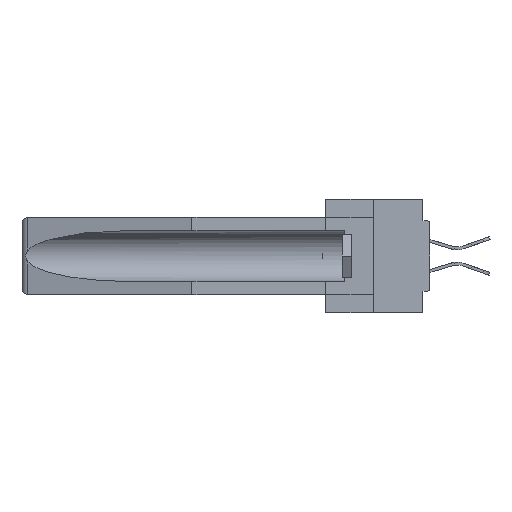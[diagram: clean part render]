
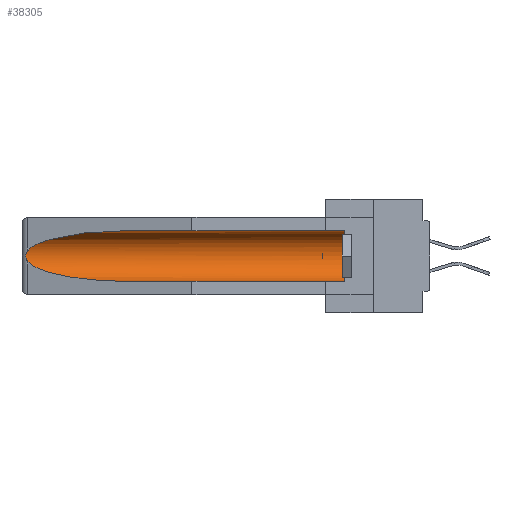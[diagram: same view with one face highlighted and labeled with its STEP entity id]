
A CAD part, left-side view. The second image highlights one B-rep face of the part: STEP entity #38305.
In plain terms, the highlighted cylindrical face has radius 2.857 mm (diameter 5.715 mm), a partial arc.
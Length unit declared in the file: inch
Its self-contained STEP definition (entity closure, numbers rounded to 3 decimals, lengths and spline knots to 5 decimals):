
#149 =( BOUNDED_CURVE ( )  B_SPLINE_CURVE ( 3, ( #30174, #41840, #18951, #27632 ),
 .UNSPECIFIED., .F., .F. ) 
 B_SPLINE_CURVE_WITH_KNOTS ( ( 4, 4 ),
 ( 4.71239, 6.08839 ),
 .UNSPECIFIED. ) 
 CURVE ( )  GEOMETRIC_REPRESENTATION_ITEM ( )  RATIONAL_B_SPLINE_CURVE ( ( 1., 0.848, 0.848, 1. ) ) 
 REPRESENTATION_ITEM ( '' )  );
#609 = VECTOR ( 'NONE', #40306, 39.37008 ) ;
#1853 = CARTESIAN_POINT ( 'NONE',  ( 0.2675, 1.53308, -0.16763 ) ) ;
#1897 = AXIS2_PLACEMENT_3D ( 'NONE', #40304, #32116, #47619 ) ;
#2174 = CARTESIAN_POINT ( 'NONE',  ( 0.26655, 1.53094, -0.18657 ) ) ;
#3349 = ORIENTED_EDGE ( 'NONE', *, *, #41865, .F. ) ;
#3635 = EDGE_CURVE ( 'NONE', #12110, #45306, #10200, .T. ) ;
#4641 = CARTESIAN_POINT ( 'NONE',  ( 0.26537, 1.52718, -0.19328 ) ) ;
#7684 = EDGE_CURVE ( 'NONE', #45306, #15028, #149, .T. ) ;
#9271 = CARTESIAN_POINT ( 'NONE',  ( 0.155, 0.126, -0.284 ) ) ;
#10200 = LINE ( 'NONE', #21074, #609 ) ;
#12110 = VERTEX_POINT ( 'NONE', #32921 ) ;
#12391 = CARTESIAN_POINT ( 'NONE',  ( 0.155, 1.07973, -0.059 ) ) ;
#13358 = CARTESIAN_POINT ( 'NONE',  ( 0.2673, 1.53269, -0.17917 ) ) ;
#13487 = DIRECTION ( 'NONE',  ( 0., 1., 0. ) ) ;
#13700 = CARTESIAN_POINT ( 'NONE',  ( 0.26597, 1.52961, -0.15275 ) ) ;
#15028 = VERTEX_POINT ( 'NONE', #18644 ) ;
#16004 = CARTESIAN_POINT ( 'NONE',  ( 0.155, -0.30754, -0.284 ) ) ;
#16397 = ORIENTED_EDGE ( 'NONE', *, *, #33899, .T. ) ;
#16442 =( BOUNDED_CURVE ( )  B_SPLINE_CURVE ( 3, ( #19342, #23220, #18688, #26744 ),
 .UNSPECIFIED., .F., .F. ) 
 B_SPLINE_CURVE_WITH_KNOTS ( ( 4, 4 ),
 ( 0.1948, 1.5708 ),
 .UNSPECIFIED. ) 
 CURVE ( )  GEOMETRIC_REPRESENTATION_ITEM ( )  RATIONAL_B_SPLINE_CURVE ( ( 1., 0.848, 0.848, 1. ) ) 
 REPRESENTATION_ITEM ( '' )  );
#17885 = ORIENTED_EDGE ( 'NONE', *, *, #40342, .T. ) ;
#18644 = CARTESIAN_POINT ( 'NONE',  ( 0.26537, 1.52718, -0.14972 ) ) ;
#18688 = CARTESIAN_POINT ( 'NONE',  ( 0.21114, 1.30732, -0.284 ) ) ;
#18951 = CARTESIAN_POINT ( 'NONE',  ( 0.25451, 1.48313, -0.09465 ) ) ;
#19236 = VERTEX_POINT ( 'NONE', #4641 ) ;
#19342 = CARTESIAN_POINT ( 'NONE',  ( 0.26537, 1.52718, -0.19328 ) ) ;
#20129 = CIRCLE ( 'NONE', #1897, 0.1125 ) ;
#21074 = CARTESIAN_POINT ( 'NONE',  ( 0.155, -0.30754, -0.059 ) ) ;
#23220 = CARTESIAN_POINT ( 'NONE',  ( 0.25451, 1.48313, -0.24835 ) ) ;
#23556 = ORIENTED_EDGE ( 'NONE', *, *, #29662, .T. ) ;
#23652 = ORIENTED_EDGE ( 'NONE', *, *, #3635, .T. ) ;
#24253 = ORIENTED_EDGE ( 'NONE', *, *, #7684, .T. ) ;
#25158 = AXIS2_PLACEMENT_3D ( 'NONE', #40441, #13487, #47932 ) ;
#26744 = CARTESIAN_POINT ( 'NONE',  ( 0.155, 1.07973, -0.284 ) ) ;
#27632 = CARTESIAN_POINT ( 'NONE',  ( 0.26537, 1.52718, -0.14972 ) ) ;
#28127 = CYLINDRICAL_SURFACE ( 'NONE', #25158, 0.1125 ) ;
#28968 = CARTESIAN_POINT ( 'NONE',  ( 0.26597, 1.5296, -0.19026 ) ) ;
#29145 = CARTESIAN_POINT ( 'NONE',  ( 0.26537, 1.52718, -0.14972 ) ) ;
#29662 = EDGE_CURVE ( 'NONE', #15028, #19236, #40975, .T. ) ;
#30119 = VECTOR ( 'NONE', #39894, 39.37008 ) ;
#30174 = CARTESIAN_POINT ( 'NONE',  ( 0.155, 1.07973, -0.059 ) ) ;
#32116 = DIRECTION ( 'NONE',  ( 0., -1., 0. ) ) ;
#32131 = EDGE_LOOP ( 'NONE', ( #24253, #23556, #17885, #3349, #16397, #23652 ) ) ;
#32295 = CARTESIAN_POINT ( 'NONE',  ( 0.26654, 1.53092, -0.15636 ) ) ;
#32668 = VERTEX_POINT ( 'NONE', #41483 ) ;
#32921 = CARTESIAN_POINT ( 'NONE',  ( 0.155, 0.126, -0.059 ) ) ;
#33899 = EDGE_CURVE ( 'NONE', #48828, #12110, #20129, .T. ) ;
#36299 = CARTESIAN_POINT ( 'NONE',  ( 0.2675, 1.53308, -0.17534 ) ) ;
#36469 = CARTESIAN_POINT ( 'NONE',  ( 0.26537, 1.52718, -0.19328 ) ) ;
#38305 = ADVANCED_FACE ( 'NONE', ( #40696 ), #28127, .F. ) ;
#39894 = DIRECTION ( 'NONE',  ( 0., 1., 0. ) ) ;
#40304 = CARTESIAN_POINT ( 'NONE',  ( 0.155, 0.126, -0.1715 ) ) ;
#40306 = DIRECTION ( 'NONE',  ( 0., 1., 0. ) ) ;
#40342 = EDGE_CURVE ( 'NONE', #19236, #32668, #16442, .T. ) ;
#40441 = CARTESIAN_POINT ( 'NONE',  ( 0.155, -0.30754, -0.1715 ) ) ;
#40696 = FACE_OUTER_BOUND ( 'NONE', #32131, .T. ) ;
#40975 = B_SPLINE_CURVE_WITH_KNOTS ( 'NONE', 3,
 ( #29145, #13700, #32295, #43803, #1853, #36299, #13358, #2174, #28968, #36469 ),
 .UNSPECIFIED., .F., .F.,
 ( 4, 2, 2, 2, 4 ),
 ( 0., 0.00029, 0.00058, 0.00087, 0.00117 ),
 .UNSPECIFIED. ) ;
#41473 = LINE ( 'NONE', #16004, #30119 ) ;
#41483 = CARTESIAN_POINT ( 'NONE',  ( 0.155, 1.07973, -0.284 ) ) ;
#41840 = CARTESIAN_POINT ( 'NONE',  ( 0.21114, 1.30732, -0.059 ) ) ;
#41865 = EDGE_CURVE ( 'NONE', #48828, #32668, #41473, .T. ) ;
#43803 = CARTESIAN_POINT ( 'NONE',  ( 0.2673, 1.5327, -0.16383 ) ) ;
#45306 = VERTEX_POINT ( 'NONE', #12391 ) ;
#47619 = DIRECTION ( 'NONE',  ( 0., 0., 1. ) ) ;
#47932 = DIRECTION ( 'NONE',  ( 0., 0., 1. ) ) ;
#48828 = VERTEX_POINT ( 'NONE', #9271 ) ;
